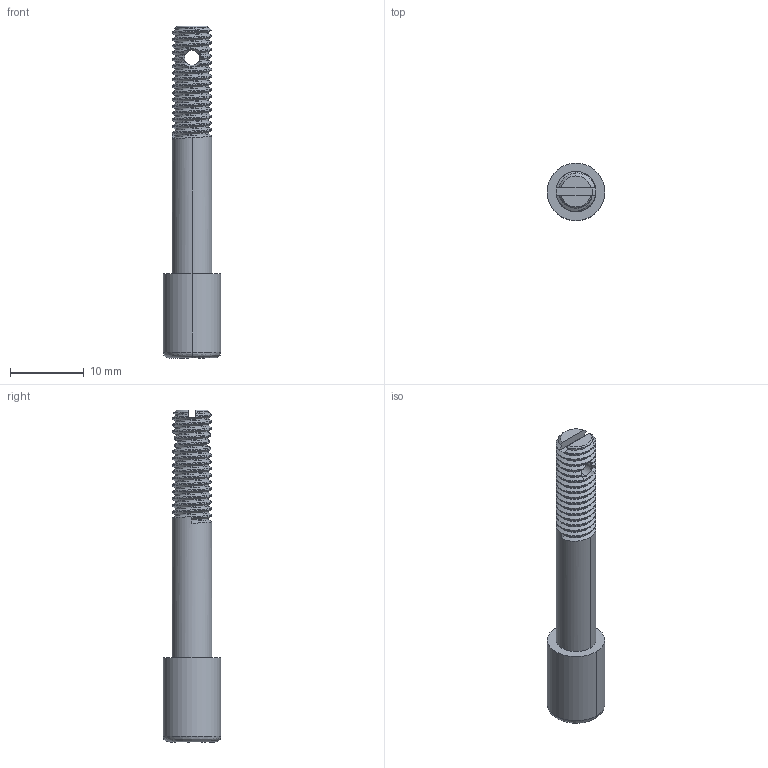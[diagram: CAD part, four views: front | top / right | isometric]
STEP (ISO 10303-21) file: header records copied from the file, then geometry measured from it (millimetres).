
FILE_DESCRIPTION (( 'STEP AP214' ), '1' );
FILE_NAME ('User Library-Telescopic Stock_Stock Bolt1.STEP', '2013-05-23T12:57:49', ( 'Asher' ), ( '' ), 'SwSTEP 2.0', 'SolidWorks 2013', '' );
FILE_SCHEMA (( 'AUTOMOTIVE_DESIGN' ));
Length unit declared in the file: millimetre
Products named in the file (1): User Library-Telescopic Stock_Stock Bolt1
Bounding box: 7.8 x 7.8 x 44.96 mm (x, y, z)
Volume: 1233.1 mm3; surface area: 1059.9 mm2
Topology: 1 solids, 1 shells, 106 faces, 309 edges, 204 vertices
Faces by surface type: cylinder 74, bspline 17, plane 8, cone 7
Entity records: 9258 total; most frequent: CARTESIAN_POINT 7025, ORIENTED_EDGE 618, EDGE_CURVE 309, DIRECTION 298, VERTEX_POINT 204, AXIS2_PLACEMENT_3D 109, EDGE_LOOP 107, FACE_OUTER_BOUND 106
